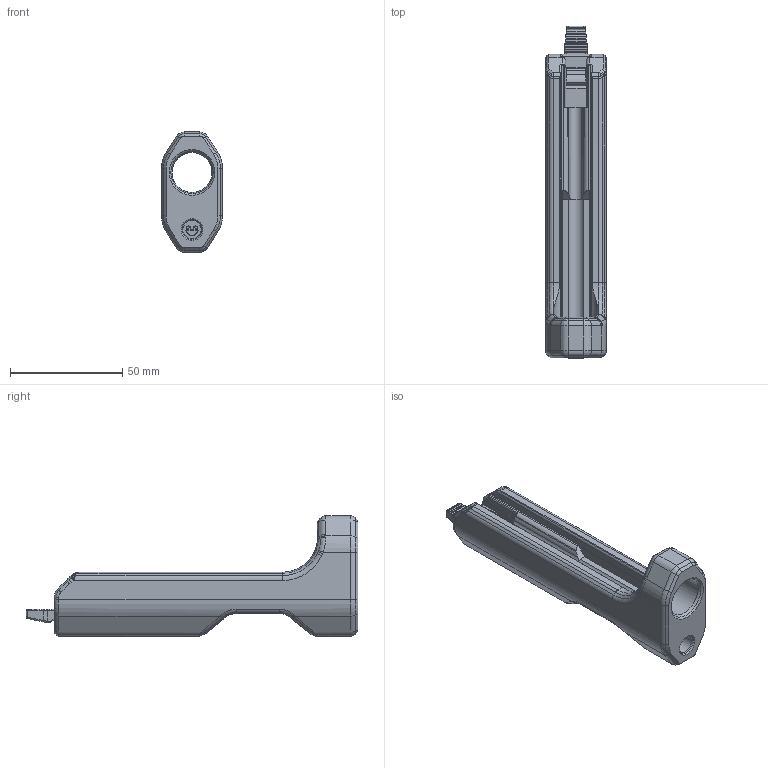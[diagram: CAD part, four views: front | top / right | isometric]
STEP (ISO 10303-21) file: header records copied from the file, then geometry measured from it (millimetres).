
FILE_DESCRIPTION(/* description */ (''),/* implementation_level */ '2;1');
FILE_NAME(/* name */ '8mm Spike Mount.step',/* time_stamp */ '2021-09-22T07:35:16-04:00',/* author */ (''),/* organization */ (''),/* preprocessor_version */ 'ST-DEVELOPER v18.1',/* originating_system */ 'Autodesk Translation Framework v10.10.0.1391',/* authorisation */ '');
FILE_SCHEMA (('AUTOMOTIVE_DESIGN { 1 0 10303 214 3 1 1 }'));
Length unit declared in the file: millimetre
Products named in the file (1): 8mm Spike
Bounding box: 27 x 147.6 x 53.45 mm (x, y, z)
Volume: 70258.9 mm3; surface area: 22523.4 mm2
Topology: 1 solids, 1 shells, 505 faces, 1247 edges, 740 vertices
Faces by surface type: cylinder 161, bspline 150, plane 112, torus 51, cone 25, sphere 6
Full cylindrical faces by diameter (mm): 8.18 x1, 17.8 x1
Entity records: 18223 total; most frequent: CARTESIAN_POINT 6992, ORIENTED_EDGE 2486, DIRECTION 2138, EDGE_CURVE 1243, AXIS2_PLACEMENT_3D 823, VERTEX_POINT 740, EDGE_LOOP 511, FACE_OUTER_BOUND 505
